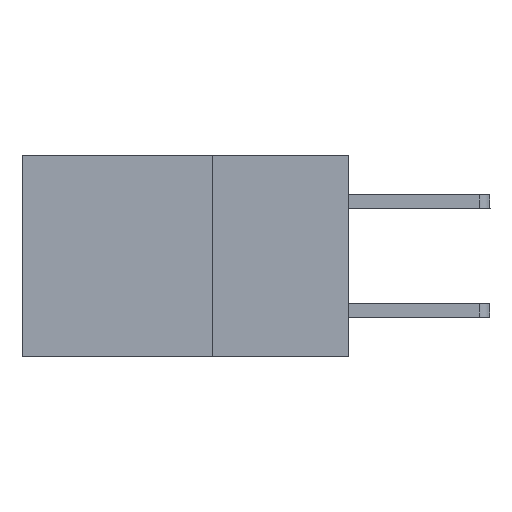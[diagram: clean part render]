
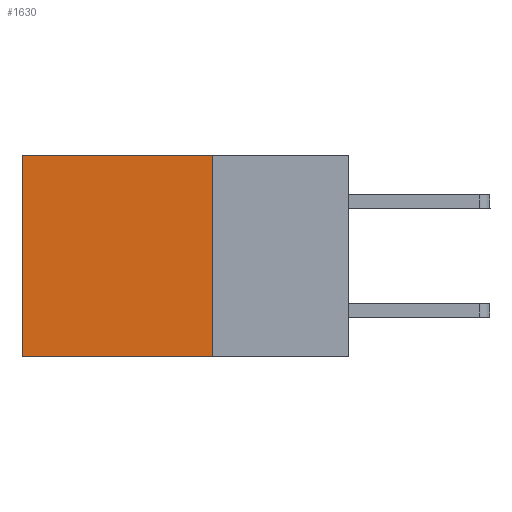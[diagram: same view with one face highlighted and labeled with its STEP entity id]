
A CAD part, left-side view. The second image highlights one B-rep face of the part: STEP entity #1630.
In plain terms, the highlighted planar face has unit normal (-1, 0, 0).
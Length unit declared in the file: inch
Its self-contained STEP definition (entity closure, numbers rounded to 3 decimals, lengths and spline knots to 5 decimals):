
#852 = ORIENTED_EDGE ( 'NONE', *, *, #1439, .T. ) ;
#851 = VERTEX_POINT ( 'NONE', #6152 ) ;
#1439 = EDGE_CURVE ( 'NONE', #1735, #9214, #5529, .T. ) ;
#1630 = ADVANCED_FACE ( 'NONE', ( #2563 ), #6776, .F. ) ;
#1735 = VERTEX_POINT ( 'NONE', #4492 ) ;
#1978 = AXIS2_PLACEMENT_3D ( 'NONE', #5751, #2730, #5954 ) ;
#2002 = CARTESIAN_POINT ( 'NONE',  ( 0.298, 0.25, 0. ) ) ;
#2102 = DIRECTION ( 'NONE',  ( 0., 0., -1. ) ) ;
#2176 = EDGE_CURVE ( 'NONE', #5435, #851, #3559, .T. ) ;
#2563 = FACE_OUTER_BOUND ( 'NONE', #9092, .T. ) ;
#2730 = DIRECTION ( 'NONE',  ( 1., 0., 0. ) ) ;
#2952 = ORIENTED_EDGE ( 'NONE', *, *, #4827, .T. ) ;
#3162 = EDGE_CURVE ( 'NONE', #851, #9214, #5225, .T. ) ;
#3559 = LINE ( 'NONE', #2002, #9638 ) ;
#3624 = DIRECTION ( 'NONE',  ( 0., 1., 0. ) ) ;
#3640 = LINE ( 'NONE', #6897, #5577 ) ;
#3978 = DIRECTION ( 'NONE',  ( 0., 0., -1. ) ) ;
#4092 = CARTESIAN_POINT ( 'NONE',  ( 0.298, 0.6, -0.37 ) ) ;
#4134 = CARTESIAN_POINT ( 'NONE',  ( 0.298, 0.25, 0. ) ) ;
#4492 = CARTESIAN_POINT ( 'NONE',  ( 0.298, 0.6, 0. ) ) ;
#4827 = EDGE_CURVE ( 'NONE', #5435, #1735, #3640, .T. ) ;
#5225 = LINE ( 'NONE', #6946, #6158 ) ;
#5298 = ORIENTED_EDGE ( 'NONE', *, *, #2176, .F. ) ;
#5435 = VERTEX_POINT ( 'NONE', #4134 ) ;
#5529 = LINE ( 'NONE', #7312, #10142 ) ;
#5577 = VECTOR ( 'NONE', #6149, 39.37008 ) ;
#5751 = CARTESIAN_POINT ( 'NONE',  ( 0.298, 0.25, 0. ) ) ;
#5954 = DIRECTION ( 'NONE',  ( 0., 0., -1. ) ) ;
#6149 = DIRECTION ( 'NONE',  ( 0., 1., 0. ) ) ;
#6152 = CARTESIAN_POINT ( 'NONE',  ( 0.298, 0.25, -0.37 ) ) ;
#6158 = VECTOR ( 'NONE', #3624, 39.37008 ) ;
#6776 = PLANE ( 'NONE',  #1978 ) ;
#6897 = CARTESIAN_POINT ( 'NONE',  ( 0.298, 0.25, 0. ) ) ;
#6946 = CARTESIAN_POINT ( 'NONE',  ( 0.298, 0.25, -0.37 ) ) ;
#7312 = CARTESIAN_POINT ( 'NONE',  ( 0.298, 0.6, 0. ) ) ;
#7785 = ORIENTED_EDGE ( 'NONE', *, *, #3162, .F. ) ;
#9092 = EDGE_LOOP ( 'NONE', ( #852, #7785, #5298, #2952 ) ) ;
#9214 = VERTEX_POINT ( 'NONE', #4092 ) ;
#9638 = VECTOR ( 'NONE', #2102, 39.37008 ) ;
#10142 = VECTOR ( 'NONE', #3978, 39.37008 ) ;
